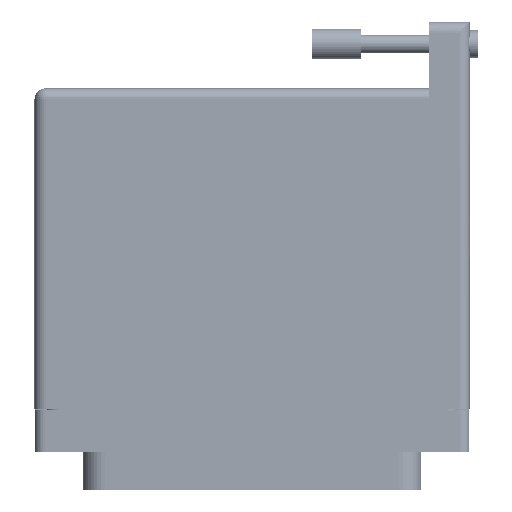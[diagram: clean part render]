
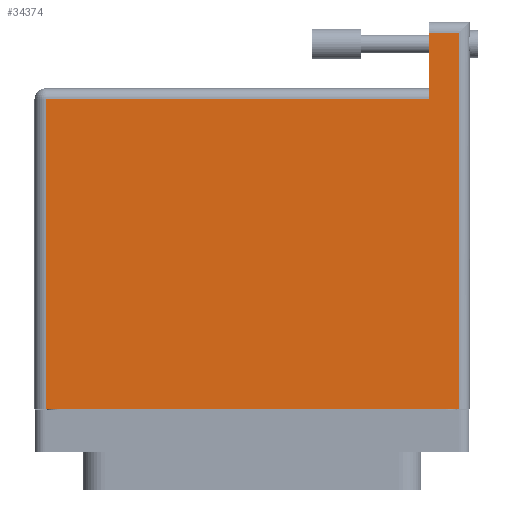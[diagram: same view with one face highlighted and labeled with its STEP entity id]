
A CAD part, front view. The second image highlights one B-rep face of the part: STEP entity #34374.
In plain terms, the highlighted face is planar.
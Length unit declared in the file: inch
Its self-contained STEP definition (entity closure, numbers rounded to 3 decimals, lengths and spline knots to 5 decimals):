
#174 = DIRECTION ( 'NONE',  ( 0., -1., 0. ) ) ;
#648 = EDGE_CURVE ( 'NONE', #63460, #43062, #47491, .T. ) ;
#1066 = LINE ( 'NONE', #17256, #45272 ) ;
#6026 = CARTESIAN_POINT ( 'NONE',  ( -1.3775, 1.93, 0.765 ) ) ;
#10065 = CARTESIAN_POINT ( 'NONE',  ( 1.3075, -0.1, 0.765 ) ) ;
#12158 = LINE ( 'NONE', #83102, #75744 ) ;
#12880 = DIRECTION ( 'NONE',  ( 0., 0., -1. ) ) ;
#15154 = VECTOR ( 'NONE', #29807, 39.37008 ) ;
#16316 = EDGE_CURVE ( 'NONE', #33087, #63460, #85188, .T. ) ;
#17256 = CARTESIAN_POINT ( 'NONE',  ( -1.3775, -0.1, 0.765 ) ) ;
#19228 = DIRECTION ( 'NONE',  ( -1., 0., 0. ) ) ;
#23971 = VERTEX_POINT ( 'NONE', #44535 ) ;
#24330 = EDGE_LOOP ( 'NONE', ( #44233, #66653, #66095, #37570, #60375, #31161 ) ) ;
#25158 = FACE_OUTER_BOUND ( 'NONE', #24330, .T. ) ;
#27505 = DIRECTION ( 'NONE',  ( 0., 1., 0. ) ) ;
#27859 = CARTESIAN_POINT ( 'NONE',  ( 1.1215, 2.28, 0.765 ) ) ;
#28264 = LINE ( 'NONE', #75376, #81007 ) ;
#29807 = DIRECTION ( 'NONE',  ( -1., 0., 0. ) ) ;
#31161 = ORIENTED_EDGE ( 'NONE', *, *, #79421, .T. ) ;
#33087 = VERTEX_POINT ( 'NONE', #27859 ) ;
#33351 = DIRECTION ( 'NONE',  ( -1., 0., 0. ) ) ;
#34374 = ADVANCED_FACE ( 'NONE', ( #25158 ), #40870, .F. ) ;
#37360 = AXIS2_PLACEMENT_3D ( 'NONE', #6026, #12880, #33351 ) ;
#37443 = CARTESIAN_POINT ( 'NONE',  ( 1.3075, 2.28, 0.765 ) ) ;
#37570 = ORIENTED_EDGE ( 'NONE', *, *, #54828, .T. ) ;
#38111 = VERTEX_POINT ( 'NONE', #37443 ) ;
#39537 = CARTESIAN_POINT ( 'NONE',  ( -1.3075, -0.1, 0.765 ) ) ;
#40870 = PLANE ( 'NONE',  #37360 ) ;
#43062 = VERTEX_POINT ( 'NONE', #85133 ) ;
#44233 = ORIENTED_EDGE ( 'NONE', *, *, #16316, .T. ) ;
#44535 = CARTESIAN_POINT ( 'NONE',  ( -1.3075, -0.1, 0.765 ) ) ;
#45272 = VECTOR ( 'NONE', #51606, 39.37008 ) ;
#47491 = LINE ( 'NONE', #57575, #15154 ) ;
#51606 = DIRECTION ( 'NONE',  ( 1., 0., 0. ) ) ;
#52763 = EDGE_CURVE ( 'NONE', #77308, #38111, #28264, .T. ) ;
#53600 = VECTOR ( 'NONE', #59783, 39.37008 ) ;
#54828 = EDGE_CURVE ( 'NONE', #23971, #77308, #1066, .T. ) ;
#57575 = CARTESIAN_POINT ( 'NONE',  ( -1.3775, 1.86, 0.765 ) ) ;
#59783 = DIRECTION ( 'NONE',  ( 0., -1., 0. ) ) ;
#60375 = ORIENTED_EDGE ( 'NONE', *, *, #52763, .T. ) ;
#61142 = LINE ( 'NONE', #39537, #53600 ) ;
#61471 = EDGE_CURVE ( 'NONE', #43062, #23971, #61142, .T. ) ;
#63460 = VERTEX_POINT ( 'NONE', #86599 ) ;
#66095 = ORIENTED_EDGE ( 'NONE', *, *, #61471, .T. ) ;
#66653 = ORIENTED_EDGE ( 'NONE', *, *, #648, .T. ) ;
#70136 = VECTOR ( 'NONE', #174, 39.37008 ) ;
#75376 = CARTESIAN_POINT ( 'NONE',  ( 1.3075, 2.35, 0.765 ) ) ;
#75744 = VECTOR ( 'NONE', #19228, 39.37008 ) ;
#77308 = VERTEX_POINT ( 'NONE', #10065 ) ;
#79421 = EDGE_CURVE ( 'NONE', #38111, #33087, #12158, .T. ) ;
#81007 = VECTOR ( 'NONE', #27505, 39.37008 ) ;
#83102 = CARTESIAN_POINT ( 'NONE',  ( -1.3775, 2.28, 0.765 ) ) ;
#83167 = CARTESIAN_POINT ( 'NONE',  ( 1.1215, 2.35, 0.765 ) ) ;
#85133 = CARTESIAN_POINT ( 'NONE',  ( -1.3075, 1.86, 0.765 ) ) ;
#85188 = LINE ( 'NONE', #83167, #70136 ) ;
#86599 = CARTESIAN_POINT ( 'NONE',  ( 1.1215, 1.86, 0.765 ) ) ;
